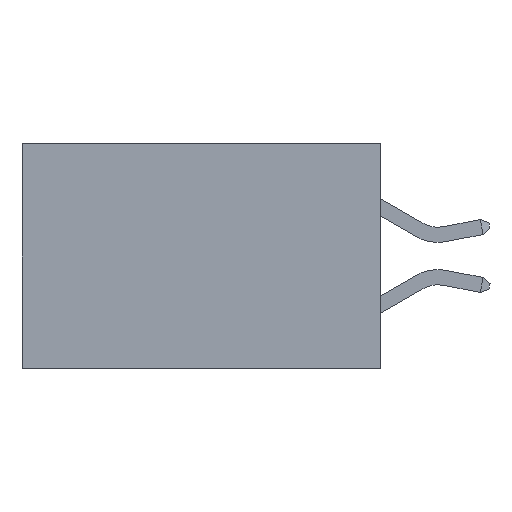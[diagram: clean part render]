
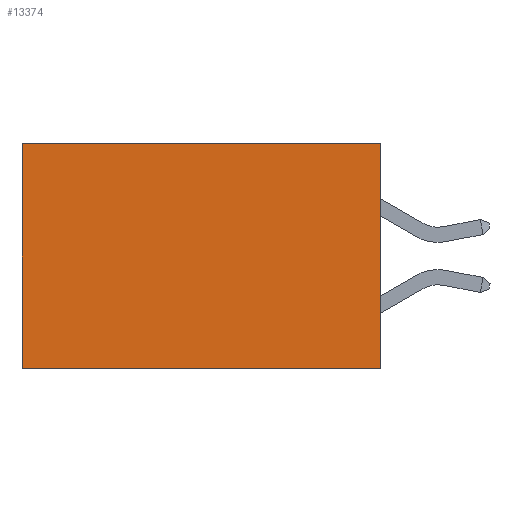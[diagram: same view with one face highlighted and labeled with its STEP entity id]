
A CAD part, left-side view. The second image highlights one B-rep face of the part: STEP entity #13374.
In plain terms, the highlighted planar face has unit normal (-1, 0, 0).
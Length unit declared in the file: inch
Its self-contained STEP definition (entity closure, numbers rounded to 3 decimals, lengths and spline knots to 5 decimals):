
#282 = LINE ( 'NONE', #26242, #12214 ) ;
#838 = CARTESIAN_POINT ( 'NONE',  ( 0.277, 0., -0.37 ) ) ;
#1006 = EDGE_CURVE ( 'NONE', #12429, #22903, #16419, .T. ) ;
#3524 = VECTOR ( 'NONE', #3705, 39.37008 ) ;
#3705 = DIRECTION ( 'NONE',  ( 0., 0., -1. ) ) ;
#3809 = EDGE_CURVE ( 'NONE', #13507, #24905, #8478, .T. ) ;
#4081 = CARTESIAN_POINT ( 'NONE',  ( 0.277, 0.59, -0.37 ) ) ;
#4146 = DIRECTION ( 'NONE',  ( 0., 1., 0. ) ) ;
#4817 = DIRECTION ( 'NONE',  ( 0., 1., 0. ) ) ;
#5125 = DIRECTION ( 'NONE',  ( 0., 0., -1. ) ) ;
#6181 = CARTESIAN_POINT ( 'NONE',  ( 0.277, 0., 0. ) ) ;
#6232 = EDGE_CURVE ( 'NONE', #22903, #24905, #9859, .T. ) ;
#8478 = LINE ( 'NONE', #15683, #20276 ) ;
#9859 = LINE ( 'NONE', #4081, #3524 ) ;
#10276 = ORIENTED_EDGE ( 'NONE', *, *, #3809, .F. ) ;
#11863 = CARTESIAN_POINT ( 'NONE',  ( 0.277, 0.59, -0.37 ) ) ;
#12214 = VECTOR ( 'NONE', #28567, 39.37008 ) ;
#12429 = VERTEX_POINT ( 'NONE', #6181 ) ;
#13374 = ADVANCED_FACE ( 'NONE', ( #25802 ), #16901, .F. ) ;
#13507 = VERTEX_POINT ( 'NONE', #838 ) ;
#14554 = CARTESIAN_POINT ( 'NONE',  ( 0.277, 0., -0.37 ) ) ;
#15682 = VECTOR ( 'NONE', #4146, 39.37008 ) ;
#15683 = CARTESIAN_POINT ( 'NONE',  ( 0.277, 0., -0.37 ) ) ;
#16419 = LINE ( 'NONE', #23659, #15682 ) ;
#16901 = PLANE ( 'NONE',  #28942 ) ;
#19275 = DIRECTION ( 'NONE',  ( 1., 0., 0. ) ) ;
#20276 = VECTOR ( 'NONE', #4817, 39.37008 ) ;
#21966 = EDGE_LOOP ( 'NONE', ( #22802, #10276, #25307, #23340 ) ) ;
#22802 = ORIENTED_EDGE ( 'NONE', *, *, #6232, .T. ) ;
#22903 = VERTEX_POINT ( 'NONE', #24941 ) ;
#23340 = ORIENTED_EDGE ( 'NONE', *, *, #1006, .T. ) ;
#23659 = CARTESIAN_POINT ( 'NONE',  ( 0.277, 0., 0. ) ) ;
#24905 = VERTEX_POINT ( 'NONE', #11863 ) ;
#24941 = CARTESIAN_POINT ( 'NONE',  ( 0.277, 0.59, 0. ) ) ;
#25307 = ORIENTED_EDGE ( 'NONE', *, *, #29894, .F. ) ;
#25802 = FACE_OUTER_BOUND ( 'NONE', #21966, .T. ) ;
#26242 = CARTESIAN_POINT ( 'NONE',  ( 0.277, 0., -0.37 ) ) ;
#28567 = DIRECTION ( 'NONE',  ( 0., 0., -1. ) ) ;
#28942 = AXIS2_PLACEMENT_3D ( 'NONE', #14554, #19275, #5125 ) ;
#29894 = EDGE_CURVE ( 'NONE', #12429, #13507, #282, .T. ) ;
